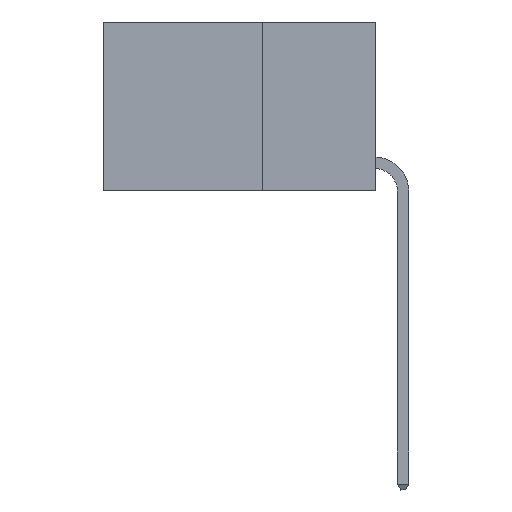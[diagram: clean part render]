
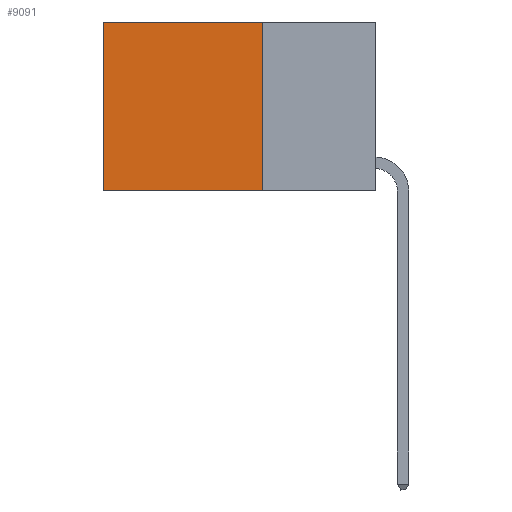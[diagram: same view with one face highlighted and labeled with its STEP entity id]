
A CAD part, left-side view. The second image highlights one B-rep face of the part: STEP entity #9091.
In plain terms, the highlighted planar face has unit normal (-1, 0, 0).
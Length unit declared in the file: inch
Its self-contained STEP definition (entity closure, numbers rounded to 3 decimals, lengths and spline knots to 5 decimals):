
#445 = AXIS2_PLACEMENT_3D ( 'NONE', #11071, #1325, #9156 ) ;
#1196 = CARTESIAN_POINT ( 'NONE',  ( 0.2625, 0.25, -0.37 ) ) ;
#1325 = DIRECTION ( 'NONE',  ( 1., 0., 0. ) ) ;
#2334 = VECTOR ( 'NONE', #15035, 39.37008 ) ;
#3231 = EDGE_CURVE ( 'NONE', #20449, #17220, #4137, .T. ) ;
#3270 = PLANE ( 'NONE',  #445 ) ;
#3271 = VECTOR ( 'NONE', #9445, 39.37008 ) ;
#3783 = VERTEX_POINT ( 'NONE', #12037 ) ;
#4137 = LINE ( 'NONE', #7985, #17687 ) ;
#4274 = ORIENTED_EDGE ( 'NONE', *, *, #18194, .F. ) ;
#4376 = ORIENTED_EDGE ( 'NONE', *, *, #3231, .T. ) ;
#4627 = DIRECTION ( 'NONE',  ( 0., 0., -1. ) ) ;
#5684 = DIRECTION ( 'NONE',  ( 0., 1., 0. ) ) ;
#6172 = EDGE_CURVE ( 'NONE', #3783, #6748, #16818, .T. ) ;
#6748 = VERTEX_POINT ( 'NONE', #24777 ) ;
#7985 = CARTESIAN_POINT ( 'NONE',  ( 0.2625, 0.25, 0. ) ) ;
#8602 = VECTOR ( 'NONE', #4627, 39.37008 ) ;
#9091 = ADVANCED_FACE ( 'NONE', ( #24971 ), #3270, .F. ) ;
#9156 = DIRECTION ( 'NONE',  ( 0., 0., -1. ) ) ;
#9347 = EDGE_LOOP ( 'NONE', ( #21639, #22737, #4274, #4376 ) ) ;
#9445 = DIRECTION ( 'NONE',  ( 0., 0., -1. ) ) ;
#11071 = CARTESIAN_POINT ( 'NONE',  ( 0.2625, 0.25, 0. ) ) ;
#11474 = CARTESIAN_POINT ( 'NONE',  ( 0.2625, 0.25, 0. ) ) ;
#11492 = LINE ( 'NONE', #13417, #3271 ) ;
#12037 = CARTESIAN_POINT ( 'NONE',  ( 0.2625, 0.25, -0.37 ) ) ;
#13417 = CARTESIAN_POINT ( 'NONE',  ( 0.2625, 0.25, 0. ) ) ;
#15035 = DIRECTION ( 'NONE',  ( 0., 1., 0. ) ) ;
#16392 = LINE ( 'NONE', #19886, #8602 ) ;
#16818 = LINE ( 'NONE', #1196, #2334 ) ;
#17220 = VERTEX_POINT ( 'NONE', #23285 ) ;
#17687 = VECTOR ( 'NONE', #5684, 39.37008 ) ;
#18194 = EDGE_CURVE ( 'NONE', #20449, #3783, #11492, .T. ) ;
#19044 = EDGE_CURVE ( 'NONE', #17220, #6748, #16392, .T. ) ;
#19886 = CARTESIAN_POINT ( 'NONE',  ( 0.2625, 0.6, 0. ) ) ;
#20449 = VERTEX_POINT ( 'NONE', #11474 ) ;
#21639 = ORIENTED_EDGE ( 'NONE', *, *, #19044, .T. ) ;
#22737 = ORIENTED_EDGE ( 'NONE', *, *, #6172, .F. ) ;
#23285 = CARTESIAN_POINT ( 'NONE',  ( 0.2625, 0.6, 0. ) ) ;
#24777 = CARTESIAN_POINT ( 'NONE',  ( 0.2625, 0.6, -0.37 ) ) ;
#24971 = FACE_OUTER_BOUND ( 'NONE', #9347, .T. ) ;
